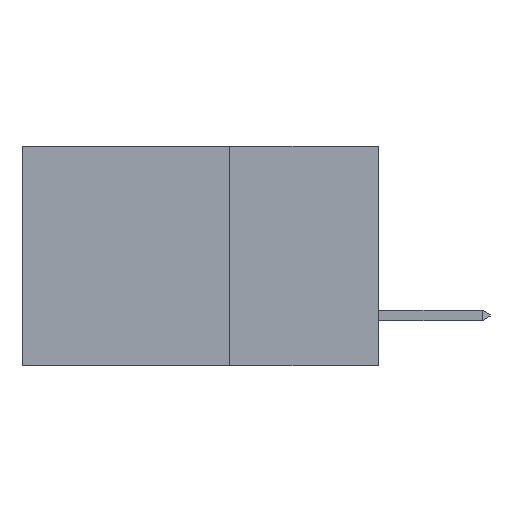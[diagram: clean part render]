
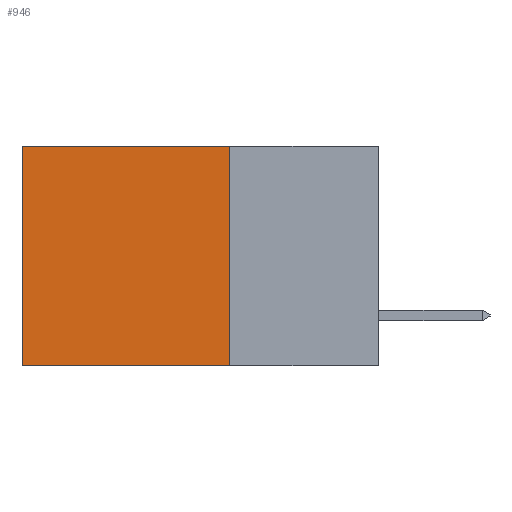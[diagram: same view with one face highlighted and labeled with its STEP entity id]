
A CAD part, left-side view. The second image highlights one B-rep face of the part: STEP entity #946.
In plain terms, the highlighted planar face has unit normal (-1, 0, 0).
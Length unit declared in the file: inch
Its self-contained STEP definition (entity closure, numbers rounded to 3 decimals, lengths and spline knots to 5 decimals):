
#15 = CARTESIAN_POINT ( 'NONE',  ( 0.2615, 0.25, 0. ) ) ;
#75 = ORIENTED_EDGE ( 'NONE', *, *, #7538, .T. ) ;
#760 = DIRECTION ( 'NONE',  ( 0., 0., -1. ) ) ;
#867 = LINE ( 'NONE', #7901, #9432 ) ;
#868 = FACE_OUTER_BOUND ( 'NONE', #1323, .T. ) ;
#946 = ADVANCED_FACE ( 'NONE', ( #868 ), #5991, .F. ) ;
#1022 = EDGE_CURVE ( 'NONE', #8962, #4474, #2613, .T. ) ;
#1142 = ORIENTED_EDGE ( 'NONE', *, *, #3027, .T. ) ;
#1323 = EDGE_LOOP ( 'NONE', ( #1142, #5063, #1437, #75 ) ) ;
#1437 = ORIENTED_EDGE ( 'NONE', *, *, #6464, .F. ) ;
#2454 = CARTESIAN_POINT ( 'NONE',  ( 0.2615, 0.6, 0. ) ) ;
#2613 = LINE ( 'NONE', #6077, #8941 ) ;
#3027 = EDGE_CURVE ( 'NONE', #5466, #4474, #9000, .T. ) ;
#3814 = CARTESIAN_POINT ( 'NONE',  ( 0.2615, 0.25, -0.37 ) ) ;
#4009 = AXIS2_PLACEMENT_3D ( 'NONE', #3814, #5993, #6042 ) ;
#4474 = VERTEX_POINT ( 'NONE', #5234 ) ;
#4639 = DIRECTION ( 'NONE',  ( 0., 0., -1. ) ) ;
#4675 = VECTOR ( 'NONE', #760, 39.37008 ) ;
#5063 = ORIENTED_EDGE ( 'NONE', *, *, #1022, .F. ) ;
#5234 = CARTESIAN_POINT ( 'NONE',  ( 0.2615, 0.6, -0.37 ) ) ;
#5466 = VERTEX_POINT ( 'NONE', #2454 ) ;
#5714 = DIRECTION ( 'NONE',  ( 0., 1., 0. ) ) ;
#5991 = PLANE ( 'NONE',  #4009 ) ;
#5993 = DIRECTION ( 'NONE',  ( 1., 0., 0. ) ) ;
#6020 = LINE ( 'NONE', #6827, #7927 ) ;
#6042 = DIRECTION ( 'NONE',  ( 0., 0., -1. ) ) ;
#6077 = CARTESIAN_POINT ( 'NONE',  ( 0.2615, 0.25, -0.37 ) ) ;
#6464 = EDGE_CURVE ( 'NONE', #10248, #8962, #867, .T. ) ;
#6827 = CARTESIAN_POINT ( 'NONE',  ( 0.2615, 0.25, 0. ) ) ;
#7538 = EDGE_CURVE ( 'NONE', #10248, #5466, #6020, .T. ) ;
#7901 = CARTESIAN_POINT ( 'NONE',  ( 0.2615, 0.25, -0.37 ) ) ;
#7927 = VECTOR ( 'NONE', #10007, 39.37008 ) ;
#8005 = CARTESIAN_POINT ( 'NONE',  ( 0.2615, 0.25, -0.37 ) ) ;
#8429 = CARTESIAN_POINT ( 'NONE',  ( 0.2615, 0.6, -0.37 ) ) ;
#8941 = VECTOR ( 'NONE', #5714, 39.37008 ) ;
#8962 = VERTEX_POINT ( 'NONE', #8005 ) ;
#9000 = LINE ( 'NONE', #8429, #4675 ) ;
#9432 = VECTOR ( 'NONE', #4639, 39.37008 ) ;
#10007 = DIRECTION ( 'NONE',  ( 0., 1., 0. ) ) ;
#10248 = VERTEX_POINT ( 'NONE', #15 ) ;
